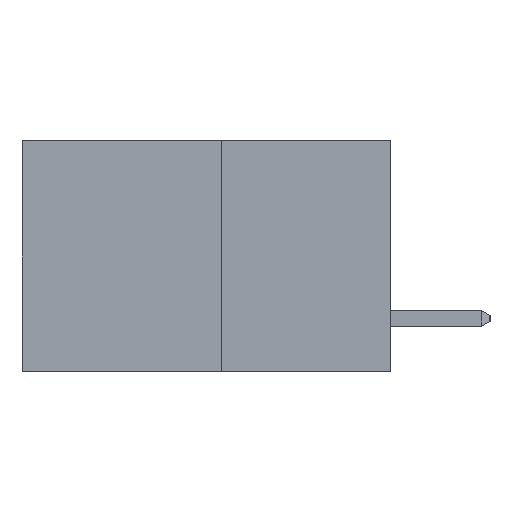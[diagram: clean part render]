
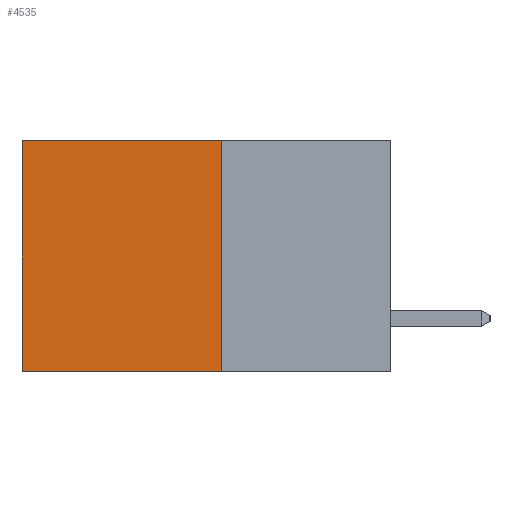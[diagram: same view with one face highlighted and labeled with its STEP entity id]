
A CAD part, left-side view. The second image highlights one B-rep face of the part: STEP entity #4535.
In plain terms, the highlighted planar face has unit normal (-1, 0, 0).
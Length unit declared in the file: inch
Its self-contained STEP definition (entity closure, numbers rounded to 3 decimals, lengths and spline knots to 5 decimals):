
#308 = DIRECTION ( 'NONE',  ( 0., 1., 0. ) ) ;
#395 = DIRECTION ( 'NONE',  ( 0., 0., -1. ) ) ;
#576 = FACE_OUTER_BOUND ( 'NONE', #13561, .T. ) ;
#847 = VECTOR ( 'NONE', #11781, 39.37008 ) ;
#1770 = ORIENTED_EDGE ( 'NONE', *, *, #14589, .F. ) ;
#2042 = CARTESIAN_POINT ( 'NONE',  ( 0.277, 0.59, -0.37 ) ) ;
#2045 = EDGE_CURVE ( 'NONE', #6599, #10343, #14125, .T. ) ;
#2651 = VECTOR ( 'NONE', #14717, 39.37008 ) ;
#3020 = DIRECTION ( 'NONE',  ( 0., 1., 0. ) ) ;
#3352 = ORIENTED_EDGE ( 'NONE', *, *, #2045, .T. ) ;
#4218 = PLANE ( 'NONE',  #12681 ) ;
#4535 = ADVANCED_FACE ( 'NONE', ( #576 ), #4218, .F. ) ;
#5340 = VERTEX_POINT ( 'NONE', #11972 ) ;
#6002 = LINE ( 'NONE', #13488, #2651 ) ;
#6368 = VERTEX_POINT ( 'NONE', #6561 ) ;
#6561 = CARTESIAN_POINT ( 'NONE',  ( 0.277, 0.27, -0.37 ) ) ;
#6599 = VERTEX_POINT ( 'NONE', #15814 ) ;
#6724 = CARTESIAN_POINT ( 'NONE',  ( 0.277, 0.27, -0.37 ) ) ;
#7961 = DIRECTION ( 'NONE',  ( 1., 0., 0. ) ) ;
#8105 = EDGE_CURVE ( 'NONE', #6368, #10343, #8318, .T. ) ;
#8249 = ORIENTED_EDGE ( 'NONE', *, *, #15988, .T. ) ;
#8318 = LINE ( 'NONE', #15207, #11259 ) ;
#10343 = VERTEX_POINT ( 'NONE', #2042 ) ;
#10600 = LINE ( 'NONE', #11731, #13485 ) ;
#11259 = VECTOR ( 'NONE', #308, 39.37008 ) ;
#11731 = CARTESIAN_POINT ( 'NONE',  ( 0.277, 0.27, 0. ) ) ;
#11781 = DIRECTION ( 'NONE',  ( 0., 0., -1. ) ) ;
#11972 = CARTESIAN_POINT ( 'NONE',  ( 0.277, 0.27, 0. ) ) ;
#12681 = AXIS2_PLACEMENT_3D ( 'NONE', #6724, #7961, #395 ) ;
#12795 = CARTESIAN_POINT ( 'NONE',  ( 0.277, 0.59, -0.37 ) ) ;
#13052 = ORIENTED_EDGE ( 'NONE', *, *, #8105, .F. ) ;
#13485 = VECTOR ( 'NONE', #3020, 39.37008 ) ;
#13488 = CARTESIAN_POINT ( 'NONE',  ( 0.277, 0.27, -0.37 ) ) ;
#13561 = EDGE_LOOP ( 'NONE', ( #3352, #13052, #1770, #8249 ) ) ;
#14125 = LINE ( 'NONE', #12795, #847 ) ;
#14589 = EDGE_CURVE ( 'NONE', #5340, #6368, #6002, .T. ) ;
#14717 = DIRECTION ( 'NONE',  ( 0., 0., -1. ) ) ;
#15207 = CARTESIAN_POINT ( 'NONE',  ( 0.277, 0.27, -0.37 ) ) ;
#15814 = CARTESIAN_POINT ( 'NONE',  ( 0.277, 0.59, 0. ) ) ;
#15988 = EDGE_CURVE ( 'NONE', #5340, #6599, #10600, .T. ) ;
